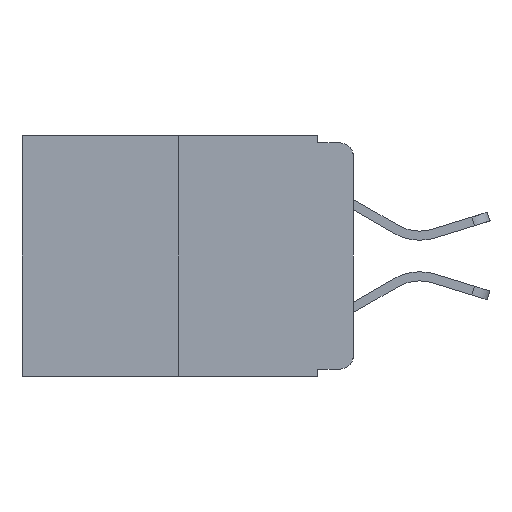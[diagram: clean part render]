
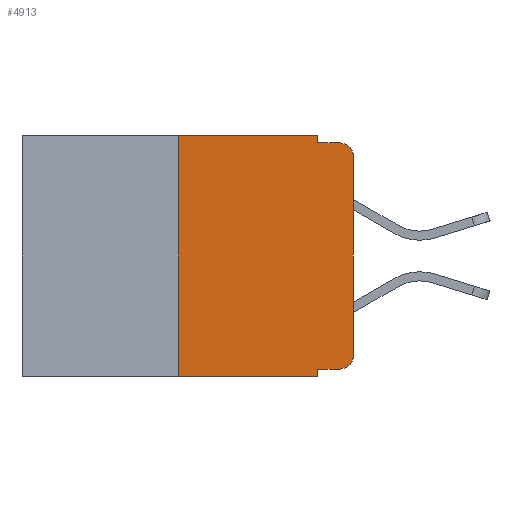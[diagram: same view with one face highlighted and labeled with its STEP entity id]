
A CAD part, left-side view. The second image highlights one B-rep face of the part: STEP entity #4913.
In plain terms, the highlighted planar face has unit normal (-1, 0, 0).
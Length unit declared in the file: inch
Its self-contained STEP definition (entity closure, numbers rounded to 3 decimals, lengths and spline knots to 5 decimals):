
#70 = CARTESIAN_POINT ( 'NONE',  ( 0., 0.051, -0.333 ) ) ;
#420 = AXIS2_PLACEMENT_3D ( 'NONE', #10754, #6973, #6988 ) ;
#445 = EDGE_CURVE ( 'NONE', #6795, #7925, #9720, .T. ) ;
#496 = CIRCLE ( 'NONE', #5505, 0.02 ) ;
#862 = LINE ( 'NONE', #4506, #9666 ) ;
#968 = VERTEX_POINT ( 'NONE', #4374 ) ;
#1095 = VERTEX_POINT ( 'NONE', #3274 ) ;
#1254 = CARTESIAN_POINT ( 'NONE',  ( 0., 0.051, -0.343 ) ) ;
#1539 = LINE ( 'NONE', #6150, #6016 ) ;
#1641 = DIRECTION ( 'NONE',  ( 0., -1., 0. ) ) ;
#2556 = EDGE_CURVE ( 'NONE', #2801, #6499, #9433, .T. ) ;
#2657 = LINE ( 'NONE', #10207, #8946 ) ;
#2801 = VERTEX_POINT ( 'NONE', #4468 ) ;
#2946 = VECTOR ( 'NONE', #5846, 39.37008 ) ;
#2950 = DIRECTION ( 'NONE',  ( 0., 0., 1. ) ) ;
#3028 = EDGE_LOOP ( 'NONE', ( #8231, #8143, #8053, #7606, #7259, #7029, #6897, #6888, #7079, #10503 ) ) ;
#3162 = DIRECTION ( 'NONE',  ( 0., 0., -1. ) ) ;
#3189 = EDGE_CURVE ( 'NONE', #1095, #6795, #8795, .T. ) ;
#3274 = CARTESIAN_POINT ( 'NONE',  ( 0., 0.051, -0.333 ) ) ;
#3275 = CARTESIAN_POINT ( 'NONE',  ( 0., 0.25, 0. ) ) ;
#3431 = EDGE_CURVE ( 'NONE', #6499, #4340, #6116, .T. ) ;
#4179 = CARTESIAN_POINT ( 'NONE',  ( 0., 0.02, -0.03 ) ) ;
#4340 = VERTEX_POINT ( 'NONE', #4745 ) ;
#4374 = CARTESIAN_POINT ( 'NONE',  ( 0., 0.02, -0.01 ) ) ;
#4468 = CARTESIAN_POINT ( 'NONE',  ( 0., 0.25, -0.343 ) ) ;
#4506 = CARTESIAN_POINT ( 'NONE',  ( 0., 0.473, -0.343 ) ) ;
#4516 = DIRECTION ( 'NONE',  ( 0., 0., -1. ) ) ;
#4589 = EDGE_CURVE ( 'NONE', #2801, #10095, #862, .T. ) ;
#4745 = CARTESIAN_POINT ( 'NONE',  ( 0., 0.051, 0. ) ) ;
#4913 = ADVANCED_FACE ( 'NONE', ( #7465 ), #6923, .F. ) ;
#5007 = DIRECTION ( 'NONE',  ( 0., 0., -1. ) ) ;
#5505 = AXIS2_PLACEMENT_3D ( 'NONE', #4179, #9726, #5007 ) ;
#5559 = AXIS2_PLACEMENT_3D ( 'NONE', #6055, #11066, #4516 ) ;
#5642 = VECTOR ( 'NONE', #2950, 39.37008 ) ;
#5846 = DIRECTION ( 'NONE',  ( 0., 0., 1. ) ) ;
#5850 = VECTOR ( 'NONE', #10521, 39.37008 ) ;
#6016 = VECTOR ( 'NONE', #9976, 39.37008 ) ;
#6055 = CARTESIAN_POINT ( 'NONE',  ( 0., 0.02, -0.313 ) ) ;
#6116 = LINE ( 'NONE', #9932, #5850 ) ;
#6150 = CARTESIAN_POINT ( 'NONE',  ( 0., 0.051, 0. ) ) ;
#6499 = VERTEX_POINT ( 'NONE', #8132 ) ;
#6515 = VECTOR ( 'NONE', #9227, 39.37008 ) ;
#6795 = VERTEX_POINT ( 'NONE', #8485 ) ;
#6888 = ORIENTED_EDGE ( 'NONE', *, *, #9879, .F. ) ;
#6897 = ORIENTED_EDGE ( 'NONE', *, *, #4589, .T. ) ;
#6923 = PLANE ( 'NONE',  #420 ) ;
#6973 = DIRECTION ( 'NONE',  ( 1., 0., 0. ) ) ;
#6988 = DIRECTION ( 'NONE',  ( 0., 0., -1. ) ) ;
#7029 = ORIENTED_EDGE ( 'NONE', *, *, #2556, .F. ) ;
#7032 = VECTOR ( 'NONE', #3162, 39.37008 ) ;
#7079 = ORIENTED_EDGE ( 'NONE', *, *, #3189, .T. ) ;
#7223 = CARTESIAN_POINT ( 'NONE',  ( 0., 0.051, 0. ) ) ;
#7259 = ORIENTED_EDGE ( 'NONE', *, *, #3431, .F. ) ;
#7465 = FACE_OUTER_BOUND ( 'NONE', #3028, .T. ) ;
#7606 = ORIENTED_EDGE ( 'NONE', *, *, #8338, .F. ) ;
#7753 = LINE ( 'NONE', #8650, #5642 ) ;
#7793 = DIRECTION ( 'NONE',  ( 0., -1., 0. ) ) ;
#7874 = CARTESIAN_POINT ( 'NONE',  ( 0., 0., -0.03 ) ) ;
#7925 = VERTEX_POINT ( 'NONE', #8329 ) ;
#8053 = ORIENTED_EDGE ( 'NONE', *, *, #9374, .F. ) ;
#8132 = CARTESIAN_POINT ( 'NONE',  ( 0., 0.25, 0. ) ) ;
#8143 = ORIENTED_EDGE ( 'NONE', *, *, #10908, .T. ) ;
#8231 = ORIENTED_EDGE ( 'NONE', *, *, #8839, .T. ) ;
#8329 = CARTESIAN_POINT ( 'NONE',  ( 0., 0., -0.313 ) ) ;
#8338 = EDGE_CURVE ( 'NONE', #4340, #8639, #8837, .T. ) ;
#8397 = CARTESIAN_POINT ( 'NONE',  ( 0., 0.051, -0.01 ) ) ;
#8485 = CARTESIAN_POINT ( 'NONE',  ( 0., 0.02, -0.333 ) ) ;
#8639 = VERTEX_POINT ( 'NONE', #8397 ) ;
#8650 = CARTESIAN_POINT ( 'NONE',  ( 0., 0., 0. ) ) ;
#8795 = LINE ( 'NONE', #70, #6515 ) ;
#8837 = LINE ( 'NONE', #7223, #7032 ) ;
#8839 = EDGE_CURVE ( 'NONE', #7925, #9755, #7753, .T. ) ;
#8946 = VECTOR ( 'NONE', #7793, 39.37008 ) ;
#9227 = DIRECTION ( 'NONE',  ( 0., -1., 0. ) ) ;
#9374 = EDGE_CURVE ( 'NONE', #8639, #968, #2657, .T. ) ;
#9433 = LINE ( 'NONE', #3275, #2946 ) ;
#9666 = VECTOR ( 'NONE', #1641, 39.37008 ) ;
#9720 = CIRCLE ( 'NONE', #5559, 0.02 ) ;
#9726 = DIRECTION ( 'NONE',  ( -1., 0., 0. ) ) ;
#9755 = VERTEX_POINT ( 'NONE', #7874 ) ;
#9879 = EDGE_CURVE ( 'NONE', #1095, #10095, #1539, .T. ) ;
#9932 = CARTESIAN_POINT ( 'NONE',  ( 0., 0.473, 0. ) ) ;
#9976 = DIRECTION ( 'NONE',  ( 0., 0., -1. ) ) ;
#10095 = VERTEX_POINT ( 'NONE', #1254 ) ;
#10207 = CARTESIAN_POINT ( 'NONE',  ( 0., 0.051, -0.01 ) ) ;
#10503 = ORIENTED_EDGE ( 'NONE', *, *, #445, .T. ) ;
#10521 = DIRECTION ( 'NONE',  ( 0., -1., 0. ) ) ;
#10754 = CARTESIAN_POINT ( 'NONE',  ( 0., 0.473, 0. ) ) ;
#10908 = EDGE_CURVE ( 'NONE', #9755, #968, #496, .T. ) ;
#11066 = DIRECTION ( 'NONE',  ( -1., 0., 0. ) ) ;
